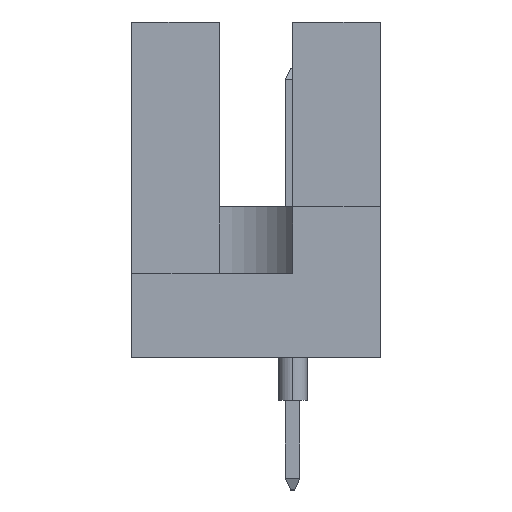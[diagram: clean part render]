
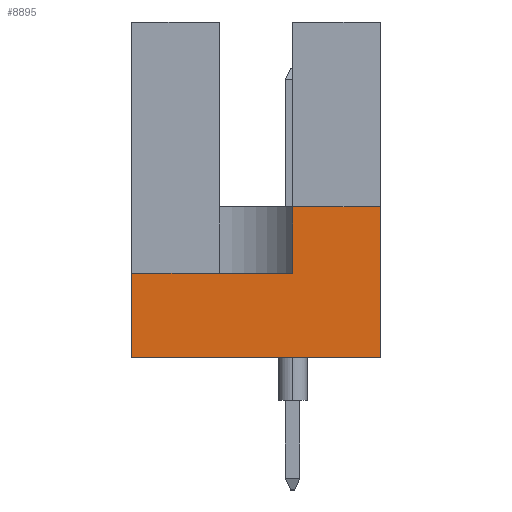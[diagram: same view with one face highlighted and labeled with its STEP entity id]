
A CAD part, left-side view. The second image highlights one B-rep face of the part: STEP entity #8895.
In plain terms, the highlighted planar face has unit normal (-1, 0, 0).
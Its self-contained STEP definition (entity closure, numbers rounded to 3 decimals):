
#64 = LINE ( 'NONE', #7523, #10365 ) ;
#369 = EDGE_CURVE ( 'NONE', #810, #6221, #11976, .T. ) ;
#409 = ORIENTED_EDGE ( 'NONE', *, *, #369, .T. ) ;
#810 = VERTEX_POINT ( 'NONE', #6149 ) ;
#1403 = CARTESIAN_POINT ( 'NONE',  ( -47.5, 4.3, 11.6 ) ) ;
#2026 = DIRECTION ( 'NONE',  ( 0., 0., -1. ) ) ;
#2245 = EDGE_CURVE ( 'NONE', #7724, #2256, #9945, .T. ) ;
#2256 = VERTEX_POINT ( 'NONE', #6150 ) ;
#2263 = DIRECTION ( 'NONE',  ( 0., -1., 0. ) ) ;
#2538 = CARTESIAN_POINT ( 'NONE',  ( -47.5, -4.3, 0. ) ) ;
#4248 = EDGE_CURVE ( 'NONE', #2256, #4395, #5237, .T. ) ;
#4395 = VERTEX_POINT ( 'NONE', #11107 ) ;
#4422 = LINE ( 'NONE', #10115, #10677 ) ;
#4683 = LINE ( 'NONE', #9274, #6171 ) ;
#5237 = LINE ( 'NONE', #9148, #5490 ) ;
#5490 = VECTOR ( 'NONE', #10998, 1000. ) ;
#5567 = VECTOR ( 'NONE', #9886, 1000. ) ;
#5758 = ORIENTED_EDGE ( 'NONE', *, *, #7543, .T. ) ;
#6036 = VERTEX_POINT ( 'NONE', #8785 ) ;
#6149 = CARTESIAN_POINT ( 'NONE',  ( -47.5, 4.3, 0. ) ) ;
#6150 = CARTESIAN_POINT ( 'NONE',  ( -47.5, -1.27, 2.9 ) ) ;
#6160 = DIRECTION ( 'NONE',  ( 0., 0., -1. ) ) ;
#6166 = DIRECTION ( 'NONE',  ( 0., -1., 0. ) ) ;
#6171 = VECTOR ( 'NONE', #2263, 1000. ) ;
#6221 = VERTEX_POINT ( 'NONE', #2538 ) ;
#6856 = AXIS2_PLACEMENT_3D ( 'NONE', #1403, #10877, #6160 ) ;
#7079 = CARTESIAN_POINT ( 'NONE',  ( -47.5, -1.27, 19.02 ) ) ;
#7409 = ORIENTED_EDGE ( 'NONE', *, *, #2245, .T. ) ;
#7523 = CARTESIAN_POINT ( 'NONE',  ( -47.5, -4.3, 11.6 ) ) ;
#7543 = EDGE_CURVE ( 'NONE', #4395, #810, #4422, .T. ) ;
#7626 = VECTOR ( 'NONE', #6166, 1000. ) ;
#7724 = VERTEX_POINT ( 'NONE', #8351 ) ;
#8025 = CARTESIAN_POINT ( 'NONE',  ( -47.5, 4.3, 0. ) ) ;
#8180 = DIRECTION ( 'NONE',  ( 0., 0., -1. ) ) ;
#8351 = CARTESIAN_POINT ( 'NONE',  ( -47.5, -1.27, 5.2 ) ) ;
#8511 = ORIENTED_EDGE ( 'NONE', *, *, #10361, .F. ) ;
#8523 = EDGE_CURVE ( 'NONE', #6036, #6221, #64, .T. ) ;
#8785 = CARTESIAN_POINT ( 'NONE',  ( -47.5, -4.3, 5.2 ) ) ;
#8895 = ADVANCED_FACE ( 'NONE', ( #10814 ), #10941, .F. ) ;
#9148 = CARTESIAN_POINT ( 'NONE',  ( -47.5, 4.3, 2.9 ) ) ;
#9274 = CARTESIAN_POINT ( 'NONE',  ( -47.5, 4.3, 5.2 ) ) ;
#9886 = DIRECTION ( 'NONE',  ( 0., 0., -1. ) ) ;
#9945 = LINE ( 'NONE', #7079, #5567 ) ;
#10036 = ORIENTED_EDGE ( 'NONE', *, *, #8523, .F. ) ;
#10115 = CARTESIAN_POINT ( 'NONE',  ( -47.5, 4.3, 11.6 ) ) ;
#10361 = EDGE_CURVE ( 'NONE', #7724, #6036, #4683, .T. ) ;
#10365 = VECTOR ( 'NONE', #2026, 1000. ) ;
#10407 = EDGE_LOOP ( 'NONE', ( #8511, #7409, #11994, #5758, #409, #10036 ) ) ;
#10677 = VECTOR ( 'NONE', #8180, 1000. ) ;
#10814 = FACE_OUTER_BOUND ( 'NONE', #10407, .T. ) ;
#10877 = DIRECTION ( 'NONE',  ( 1., 0., 0. ) ) ;
#10941 = PLANE ( 'NONE',  #6856 ) ;
#10998 = DIRECTION ( 'NONE',  ( 0., 1., 0. ) ) ;
#11107 = CARTESIAN_POINT ( 'NONE',  ( -47.5, 4.3, 2.9 ) ) ;
#11976 = LINE ( 'NONE', #8025, #7626 ) ;
#11994 = ORIENTED_EDGE ( 'NONE', *, *, #4248, .T. ) ;
